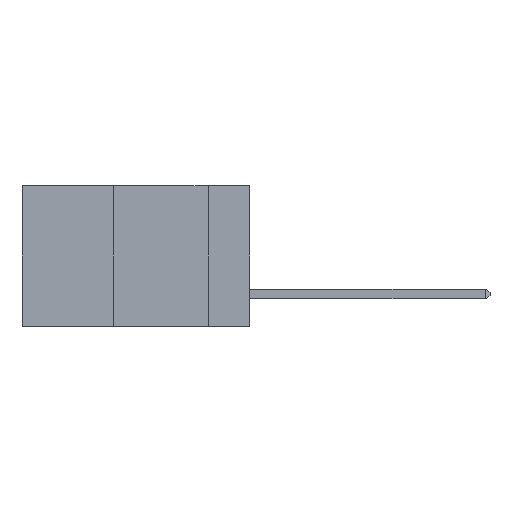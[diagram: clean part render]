
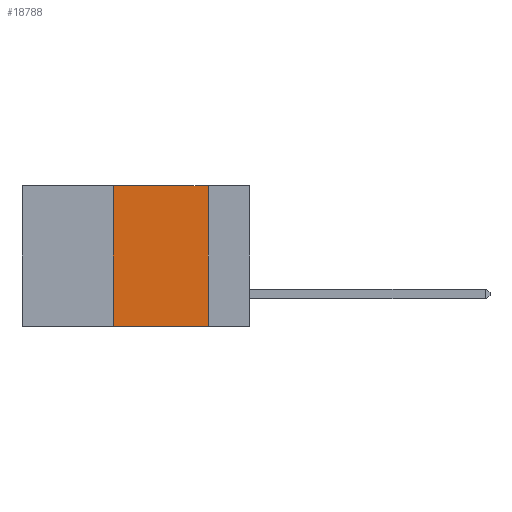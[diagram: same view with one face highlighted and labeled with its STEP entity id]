
A CAD part, left-side view. The second image highlights one B-rep face of the part: STEP entity #18788.
In plain terms, the highlighted planar face has unit normal (-1, 0, 0).
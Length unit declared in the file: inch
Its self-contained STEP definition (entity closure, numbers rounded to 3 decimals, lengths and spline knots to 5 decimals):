
#1346 = CARTESIAN_POINT ( 'NONE',  ( 0., 0.36, -0.37 ) ) ;
#4093 = CARTESIAN_POINT ( 'NONE',  ( 0., 0.6, 0. ) ) ;
#4310 = EDGE_CURVE ( 'NONE', #27735, #30428, #22759, .T. ) ;
#4524 = ORIENTED_EDGE ( 'NONE', *, *, #24969, .F. ) ;
#5161 = AXIS2_PLACEMENT_3D ( 'NONE', #24359, #31705, #17123 ) ;
#5608 = LINE ( 'NONE', #28853, #17200 ) ;
#6182 = VECTOR ( 'NONE', #11521, 39.37008 ) ;
#6717 = EDGE_CURVE ( 'NONE', #27735, #14599, #19173, .T. ) ;
#7512 = CARTESIAN_POINT ( 'NONE',  ( 0., 0.36, 0. ) ) ;
#7673 = VERTEX_POINT ( 'NONE', #18175 ) ;
#8850 = VECTOR ( 'NONE', #27238, 39.37008 ) ;
#9800 = CARTESIAN_POINT ( 'NONE',  ( 0., 0.11, -0.37 ) ) ;
#11521 = DIRECTION ( 'NONE',  ( 0., -1., 0. ) ) ;
#12623 = VECTOR ( 'NONE', #14362, 39.37008 ) ;
#13536 = LINE ( 'NONE', #4093, #6182 ) ;
#14362 = DIRECTION ( 'NONE',  ( 0., -1., 0. ) ) ;
#14599 = VERTEX_POINT ( 'NONE', #9800 ) ;
#14961 = FACE_OUTER_BOUND ( 'NONE', #22757, .T. ) ;
#17123 = DIRECTION ( 'NONE',  ( 0., 0., -1. ) ) ;
#17200 = VECTOR ( 'NONE', #31302, 39.37008 ) ;
#18175 = CARTESIAN_POINT ( 'NONE',  ( 0., 0.11, 0. ) ) ;
#18788 = ADVANCED_FACE ( 'NONE', ( #14961 ), #29255, .F. ) ;
#19173 = LINE ( 'NONE', #24073, #12623 ) ;
#19185 = ORIENTED_EDGE ( 'NONE', *, *, #6717, .T. ) ;
#22757 = EDGE_LOOP ( 'NONE', ( #23364, #4524, #31355, #19185 ) ) ;
#22759 = LINE ( 'NONE', #24757, #8850 ) ;
#23364 = ORIENTED_EDGE ( 'NONE', *, *, #27879, .F. ) ;
#24073 = CARTESIAN_POINT ( 'NONE',  ( 0., 0.6, -0.37 ) ) ;
#24359 = CARTESIAN_POINT ( 'NONE',  ( 0., 0.6, 0. ) ) ;
#24757 = CARTESIAN_POINT ( 'NONE',  ( 0., 0.36, 0. ) ) ;
#24969 = EDGE_CURVE ( 'NONE', #30428, #7673, #13536, .T. ) ;
#27238 = DIRECTION ( 'NONE',  ( 0., 0., 1. ) ) ;
#27735 = VERTEX_POINT ( 'NONE', #1346 ) ;
#27879 = EDGE_CURVE ( 'NONE', #7673, #14599, #5608, .T. ) ;
#28853 = CARTESIAN_POINT ( 'NONE',  ( 0., 0.11, 0. ) ) ;
#29255 = PLANE ( 'NONE',  #5161 ) ;
#30428 = VERTEX_POINT ( 'NONE', #7512 ) ;
#31302 = DIRECTION ( 'NONE',  ( 0., 0., -1. ) ) ;
#31355 = ORIENTED_EDGE ( 'NONE', *, *, #4310, .F. ) ;
#31705 = DIRECTION ( 'NONE',  ( 1., 0., 0. ) ) ;
